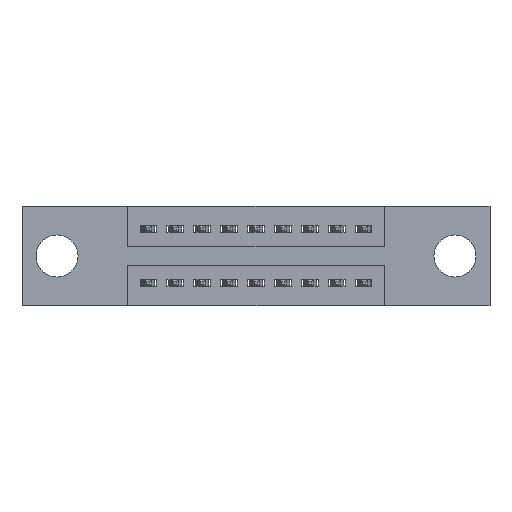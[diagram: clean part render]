
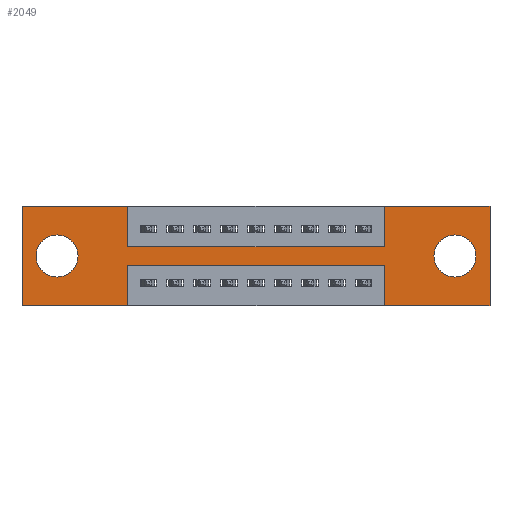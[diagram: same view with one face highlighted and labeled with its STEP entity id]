
A CAD part, front view. The second image highlights one B-rep face of the part: STEP entity #2049.
In plain terms, the highlighted planar face has unit normal (0, -1, 0).
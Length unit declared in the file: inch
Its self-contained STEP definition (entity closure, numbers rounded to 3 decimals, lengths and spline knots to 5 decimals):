
#197 = EDGE_CURVE ( 'NONE', #5665, #305, #4362, .T. ) ;
#206 = AXIS2_PLACEMENT_3D ( 'NONE', #10944, #2660, #1878 ) ;
#301 = CARTESIAN_POINT ( 'NONE',  ( 0.3925, 0., -0.22 ) ) ;
#305 = VERTEX_POINT ( 'NONE', #1291 ) ;
#346 = DIRECTION ( 'NONE',  ( 1., 0., 0. ) ) ;
#385 = EDGE_CURVE ( 'NONE', #2649, #1362, #7969, .T. ) ;
#495 = CARTESIAN_POINT ( 'NONE',  ( 0., 0., 0. ) ) ;
#496 = ORIENTED_EDGE ( 'NONE', *, *, #5598, .F. ) ;
#620 = ORIENTED_EDGE ( 'NONE', *, *, #11148, .F. ) ;
#727 = VERTEX_POINT ( 'NONE', #3204 ) ;
#728 = VERTEX_POINT ( 'NONE', #10580 ) ;
#730 = DIRECTION ( 'NONE',  ( 0., 0., -1. ) ) ;
#752 = AXIS2_PLACEMENT_3D ( 'NONE', #3950, #5479, #7641 ) ;
#827 = ORIENTED_EDGE ( 'NONE', *, *, #3903, .F. ) ;
#840 = DIRECTION ( 'NONE',  ( 0., 0., -1. ) ) ;
#895 = CARTESIAN_POINT ( 'NONE',  ( 0.13, 0., -0.185 ) ) ;
#1019 = ORIENTED_EDGE ( 'NONE', *, *, #197, .T. ) ;
#1113 = DIRECTION ( 'NONE',  ( 0., 0., 1. ) ) ;
#1146 = CARTESIAN_POINT ( 'NONE',  ( 0.13, 0., -0.263 ) ) ;
#1251 = VECTOR ( 'NONE', #1113, 39.37008 ) ;
#1291 = CARTESIAN_POINT ( 'NONE',  ( 0.13, 0., -0.107 ) ) ;
#1362 = VERTEX_POINT ( 'NONE', #7257 ) ;
#1375 = VECTOR ( 'NONE', #5069, 39.37008 ) ;
#1517 = EDGE_CURVE ( 'NONE', #8023, #8321, #6029, .T. ) ;
#1674 = LINE ( 'NONE', #11168, #3673 ) ;
#1783 = FACE_OUTER_BOUND ( 'NONE', #3789, .T. ) ;
#1784 = CARTESIAN_POINT ( 'NONE',  ( 1.605, 0., -0.107 ) ) ;
#1870 = VERTEX_POINT ( 'NONE', #5551 ) ;
#1878 = DIRECTION ( 'NONE',  ( 0., 0., 1. ) ) ;
#1958 = VERTEX_POINT ( 'NONE', #10350 ) ;
#1993 = CARTESIAN_POINT ( 'NONE',  ( 1.605, 0., -0.185 ) ) ;
#2049 = ADVANCED_FACE ( 'NONE', ( #2124, #3668, #1783 ), #7425, .T. ) ;
#2089 = DIRECTION ( 'NONE',  ( 0., 0., 1. ) ) ;
#2092 = CARTESIAN_POINT ( 'NONE',  ( 0.3925, 0., -0.37 ) ) ;
#2097 = CARTESIAN_POINT ( 'NONE',  ( 0.3925, 0., -0.15 ) ) ;
#2124 = FACE_BOUND ( 'NONE', #6219, .T. ) ;
#2405 = CARTESIAN_POINT ( 'NONE',  ( 1.3425, 0., 0. ) ) ;
#2438 = DIRECTION ( 'NONE',  ( 0., 0., 1. ) ) ;
#2611 = VECTOR ( 'NONE', #346, 39.37008 ) ;
#2649 = VERTEX_POINT ( 'NONE', #7997 ) ;
#2660 = DIRECTION ( 'NONE',  ( 0., 1., 0. ) ) ;
#2827 = CARTESIAN_POINT ( 'NONE',  ( 1.735, 0., 0. ) ) ;
#3006 = EDGE_CURVE ( 'NONE', #728, #8454, #5845, .T. ) ;
#3032 = ORIENTED_EDGE ( 'NONE', *, *, #5535, .T. ) ;
#3045 = LINE ( 'NONE', #495, #4257 ) ;
#3145 = ORIENTED_EDGE ( 'NONE', *, *, #1517, .T. ) ;
#3204 = CARTESIAN_POINT ( 'NONE',  ( 0.3925, 0., -0.22 ) ) ;
#3399 = ORIENTED_EDGE ( 'NONE', *, *, #3006, .F. ) ;
#3444 = VECTOR ( 'NONE', #5790, 39.37008 ) ;
#3523 = LINE ( 'NONE', #5101, #5968 ) ;
#3549 = AXIS2_PLACEMENT_3D ( 'NONE', #1993, #9148, #840 ) ;
#3613 = EDGE_CURVE ( 'NONE', #11317, #1870, #3523, .T. ) ;
#3668 = FACE_BOUND ( 'NONE', #8631, .T. ) ;
#3673 = VECTOR ( 'NONE', #6699, 39.37008 ) ;
#3700 = CIRCLE ( 'NONE', #206, 0.078 ) ;
#3703 = LINE ( 'NONE', #11074, #8538 ) ;
#3753 = CIRCLE ( 'NONE', #3549, 0.078 ) ;
#3789 = EDGE_LOOP ( 'NONE', ( #10933, #827, #8466, #11156, #9756, #5686, #11873, #3399, #496, #620, #4569, #11146 ) ) ;
#3903 = EDGE_CURVE ( 'NONE', #1362, #727, #4911, .T. ) ;
#3950 = CARTESIAN_POINT ( 'NONE',  ( 0., 0., -0.37 ) ) ;
#4001 = DIRECTION ( 'NONE',  ( -1., 0., 0. ) ) ;
#4038 = DIRECTION ( 'NONE',  ( 0., 1., 0. ) ) ;
#4122 = EDGE_CURVE ( 'NONE', #1870, #2649, #1674, .T. ) ;
#4257 = VECTOR ( 'NONE', #10536, 39.37008 ) ;
#4362 = CIRCLE ( 'NONE', #6488, 0.078 ) ;
#4569 = ORIENTED_EDGE ( 'NONE', *, *, #10706, .F. ) ;
#4594 = DIRECTION ( 'NONE',  ( 0., 1., 0. ) ) ;
#4647 = CARTESIAN_POINT ( 'NONE',  ( 1.3425, 0., 0. ) ) ;
#4781 = EDGE_CURVE ( 'NONE', #9544, #11317, #3045, .T. ) ;
#4801 = CARTESIAN_POINT ( 'NONE',  ( 0., 0., 0. ) ) ;
#4890 = CARTESIAN_POINT ( 'NONE',  ( 1.605, 0., -0.185 ) ) ;
#4911 = LINE ( 'NONE', #301, #7929 ) ;
#4951 = VERTEX_POINT ( 'NONE', #11689 ) ;
#5069 = DIRECTION ( 'NONE',  ( 0., 0., 1. ) ) ;
#5101 = CARTESIAN_POINT ( 'NONE',  ( 1.735, 0., 0. ) ) ;
#5207 = CARTESIAN_POINT ( 'NONE',  ( 0.3925, 0., 0. ) ) ;
#5431 = VERTEX_POINT ( 'NONE', #5207 ) ;
#5479 = DIRECTION ( 'NONE',  ( 0., -1., 0. ) ) ;
#5535 = EDGE_CURVE ( 'NONE', #305, #5665, #3700, .T. ) ;
#5551 = CARTESIAN_POINT ( 'NONE',  ( 1.735, 0., -0.37 ) ) ;
#5553 = CARTESIAN_POINT ( 'NONE',  ( 0., 0., -0.37 ) ) ;
#5598 = EDGE_CURVE ( 'NONE', #5431, #728, #3703, .T. ) ;
#5665 = VERTEX_POINT ( 'NONE', #1146 ) ;
#5686 = ORIENTED_EDGE ( 'NONE', *, *, #4781, .F. ) ;
#5713 = LINE ( 'NONE', #4801, #1251 ) ;
#5790 = DIRECTION ( 'NONE',  ( 1., 0., 0. ) ) ;
#5826 = EDGE_CURVE ( 'NONE', #8454, #9544, #7006, .T. ) ;
#5845 = LINE ( 'NONE', #2097, #3444 ) ;
#5968 = VECTOR ( 'NONE', #730, 39.37008 ) ;
#6029 = CIRCLE ( 'NONE', #6799, 0.078 ) ;
#6030 = DIRECTION ( 'NONE',  ( 0., 0., -1. ) ) ;
#6219 = EDGE_LOOP ( 'NONE', ( #3145, #8677 ) ) ;
#6488 = AXIS2_PLACEMENT_3D ( 'NONE', #895, #4594, #2089 ) ;
#6699 = DIRECTION ( 'NONE',  ( -1., 0., 0. ) ) ;
#6799 = AXIS2_PLACEMENT_3D ( 'NONE', #4890, #4038, #6030 ) ;
#7006 = LINE ( 'NONE', #2405, #1375 ) ;
#7046 = CARTESIAN_POINT ( 'NONE',  ( 0.3925, 0., -0.37 ) ) ;
#7061 = VECTOR ( 'NONE', #7554, 39.37008 ) ;
#7257 = CARTESIAN_POINT ( 'NONE',  ( 1.3425, 0., -0.22 ) ) ;
#7425 = PLANE ( 'NONE',  #752 ) ;
#7554 = DIRECTION ( 'NONE',  ( -1., 0., 0. ) ) ;
#7614 = DIRECTION ( 'NONE',  ( 0., 0., -1. ) ) ;
#7641 = DIRECTION ( 'NONE',  ( 0., 0., -1. ) ) ;
#7802 = EDGE_CURVE ( 'NONE', #8321, #8023, #3753, .T. ) ;
#7929 = VECTOR ( 'NONE', #4001, 39.37008 ) ;
#7969 = LINE ( 'NONE', #11636, #11538 ) ;
#7997 = CARTESIAN_POINT ( 'NONE',  ( 1.3425, 0., -0.37 ) ) ;
#8023 = VERTEX_POINT ( 'NONE', #1784 ) ;
#8321 = VERTEX_POINT ( 'NONE', #9103 ) ;
#8443 = VECTOR ( 'NONE', #7614, 39.37008 ) ;
#8454 = VERTEX_POINT ( 'NONE', #9938 ) ;
#8466 = ORIENTED_EDGE ( 'NONE', *, *, #385, .F. ) ;
#8538 = VECTOR ( 'NONE', #10225, 39.37008 ) ;
#8631 = EDGE_LOOP ( 'NONE', ( #3032, #1019 ) ) ;
#8677 = ORIENTED_EDGE ( 'NONE', *, *, #7802, .T. ) ;
#9103 = CARTESIAN_POINT ( 'NONE',  ( 1.605, 0., -0.263 ) ) ;
#9148 = DIRECTION ( 'NONE',  ( 0., 1., 0. ) ) ;
#9544 = VERTEX_POINT ( 'NONE', #4647 ) ;
#9734 = CARTESIAN_POINT ( 'NONE',  ( 0., 0., 0. ) ) ;
#9756 = ORIENTED_EDGE ( 'NONE', *, *, #3613, .F. ) ;
#9938 = CARTESIAN_POINT ( 'NONE',  ( 1.3425, 0., -0.15 ) ) ;
#10225 = DIRECTION ( 'NONE',  ( 0., 0., -1. ) ) ;
#10350 = CARTESIAN_POINT ( 'NONE',  ( 0., 0., -0.37 ) ) ;
#10376 = LINE ( 'NONE', #2092, #8443 ) ;
#10411 = VERTEX_POINT ( 'NONE', #7046 ) ;
#10536 = DIRECTION ( 'NONE',  ( 1., 0., 0. ) ) ;
#10580 = CARTESIAN_POINT ( 'NONE',  ( 0.3925, 0., -0.15 ) ) ;
#10706 = EDGE_CURVE ( 'NONE', #1958, #4951, #5713, .T. ) ;
#10933 = ORIENTED_EDGE ( 'NONE', *, *, #11497, .F. ) ;
#10944 = CARTESIAN_POINT ( 'NONE',  ( 0.13, 0., -0.185 ) ) ;
#11074 = CARTESIAN_POINT ( 'NONE',  ( 0.3925, 0., 0. ) ) ;
#11146 = ORIENTED_EDGE ( 'NONE', *, *, #11286, .F. ) ;
#11148 = EDGE_CURVE ( 'NONE', #4951, #5431, #11541, .T. ) ;
#11156 = ORIENTED_EDGE ( 'NONE', *, *, #4122, .F. ) ;
#11168 = CARTESIAN_POINT ( 'NONE',  ( 0., 0., -0.37 ) ) ;
#11286 = EDGE_CURVE ( 'NONE', #10411, #1958, #11957, .T. ) ;
#11317 = VERTEX_POINT ( 'NONE', #2827 ) ;
#11497 = EDGE_CURVE ( 'NONE', #727, #10411, #10376, .T. ) ;
#11538 = VECTOR ( 'NONE', #2438, 39.37008 ) ;
#11541 = LINE ( 'NONE', #9734, #2611 ) ;
#11636 = CARTESIAN_POINT ( 'NONE',  ( 1.3425, 0., -0.37 ) ) ;
#11689 = CARTESIAN_POINT ( 'NONE',  ( 0., 0., 0. ) ) ;
#11873 = ORIENTED_EDGE ( 'NONE', *, *, #5826, .F. ) ;
#11957 = LINE ( 'NONE', #5553, #7061 ) ;
